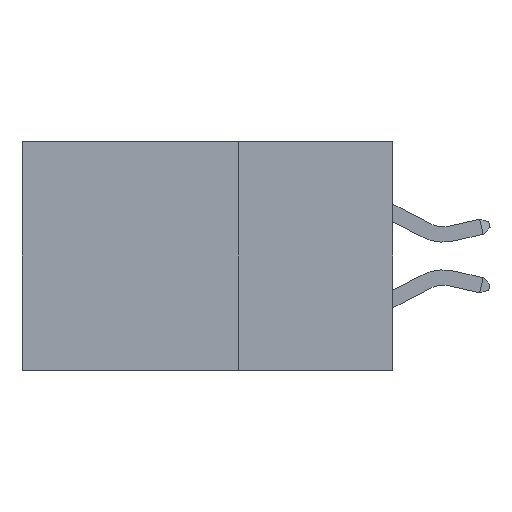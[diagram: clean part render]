
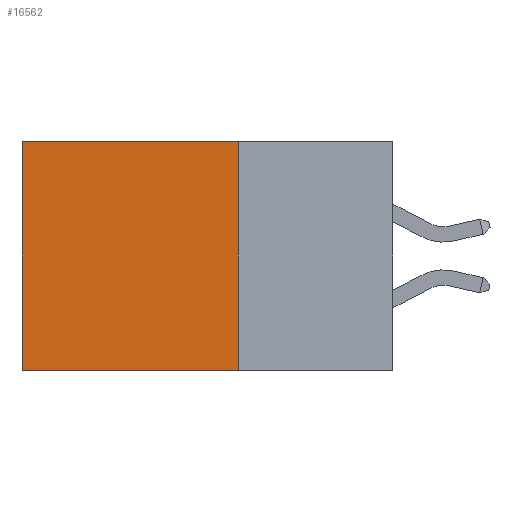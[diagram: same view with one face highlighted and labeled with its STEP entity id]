
A CAD part, left-side view. The second image highlights one B-rep face of the part: STEP entity #16562.
In plain terms, the highlighted planar face has unit normal (-1, 0, 0).
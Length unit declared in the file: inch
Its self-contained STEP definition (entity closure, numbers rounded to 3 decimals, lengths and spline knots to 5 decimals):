
#614 = FACE_OUTER_BOUND ( 'NONE', #5682, .T. ) ;
#2354 = VECTOR ( 'NONE', #8761, 39.37008 ) ;
#3647 = EDGE_CURVE ( 'NONE', #6958, #8651, #34931, .T. ) ;
#4669 = CARTESIAN_POINT ( 'NONE',  ( 0.2875, 0.25, -0.37 ) ) ;
#5682 = EDGE_LOOP ( 'NONE', ( #28806, #15920, #37246, #12543 ) ) ;
#6633 = DIRECTION ( 'NONE',  ( 1., 0., 0. ) ) ;
#6958 = VERTEX_POINT ( 'NONE', #28795 ) ;
#7131 = DIRECTION ( 'NONE',  ( 0., 0., -1. ) ) ;
#8651 = VERTEX_POINT ( 'NONE', #29978 ) ;
#8761 = DIRECTION ( 'NONE',  ( 0., 1., 0. ) ) ;
#9492 = EDGE_CURVE ( 'NONE', #18722, #12570, #16612, .T. ) ;
#10343 = CARTESIAN_POINT ( 'NONE',  ( 0.2875, 0.25, 0. ) ) ;
#12543 = ORIENTED_EDGE ( 'NONE', *, *, #3647, .T. ) ;
#12570 = VERTEX_POINT ( 'NONE', #16403 ) ;
#14141 = DIRECTION ( 'NONE',  ( 0., 0., -1. ) ) ;
#14543 = VECTOR ( 'NONE', #34596, 39.37008 ) ;
#15920 = ORIENTED_EDGE ( 'NONE', *, *, #9492, .F. ) ;
#16403 = CARTESIAN_POINT ( 'NONE',  ( 0.2875, 0.6, -0.37 ) ) ;
#16461 = CARTESIAN_POINT ( 'NONE',  ( 0.2875, 0.25, 0. ) ) ;
#16562 = ADVANCED_FACE ( 'NONE', ( #614 ), #30306, .F. ) ;
#16612 = LINE ( 'NONE', #4669, #21848 ) ;
#18433 = CARTESIAN_POINT ( 'NONE',  ( 0.2875, 0.25, 0. ) ) ;
#18722 = VERTEX_POINT ( 'NONE', #42621 ) ;
#21848 = VECTOR ( 'NONE', #29350, 39.37008 ) ;
#23149 = VECTOR ( 'NONE', #7131, 39.37008 ) ;
#26719 = EDGE_CURVE ( 'NONE', #6958, #18722, #41308, .T. ) ;
#28795 = CARTESIAN_POINT ( 'NONE',  ( 0.2875, 0.25, 0. ) ) ;
#28806 = ORIENTED_EDGE ( 'NONE', *, *, #42795, .T. ) ;
#29350 = DIRECTION ( 'NONE',  ( 0., 1., 0. ) ) ;
#29978 = CARTESIAN_POINT ( 'NONE',  ( 0.2875, 0.6, 0. ) ) ;
#30306 = PLANE ( 'NONE',  #40942 ) ;
#34596 = DIRECTION ( 'NONE',  ( 0., 0., -1. ) ) ;
#34931 = LINE ( 'NONE', #18433, #2354 ) ;
#35034 = CARTESIAN_POINT ( 'NONE',  ( 0.2875, 0.6, 0. ) ) ;
#37246 = ORIENTED_EDGE ( 'NONE', *, *, #26719, .F. ) ;
#40942 = AXIS2_PLACEMENT_3D ( 'NONE', #16461, #6633, #14141 ) ;
#40956 = LINE ( 'NONE', #35034, #14543 ) ;
#41308 = LINE ( 'NONE', #10343, #23149 ) ;
#42621 = CARTESIAN_POINT ( 'NONE',  ( 0.2875, 0.25, -0.37 ) ) ;
#42795 = EDGE_CURVE ( 'NONE', #8651, #12570, #40956, .T. ) ;
